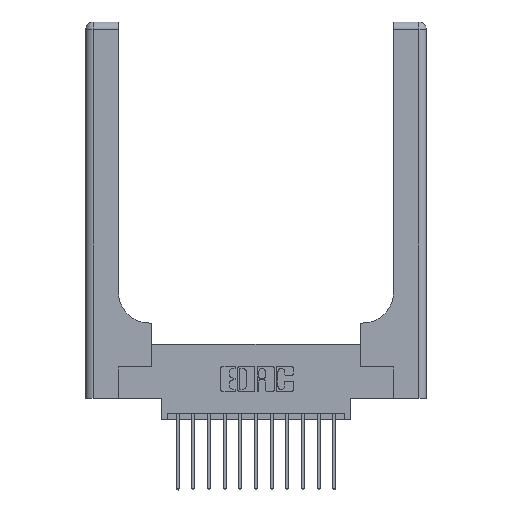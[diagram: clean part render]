
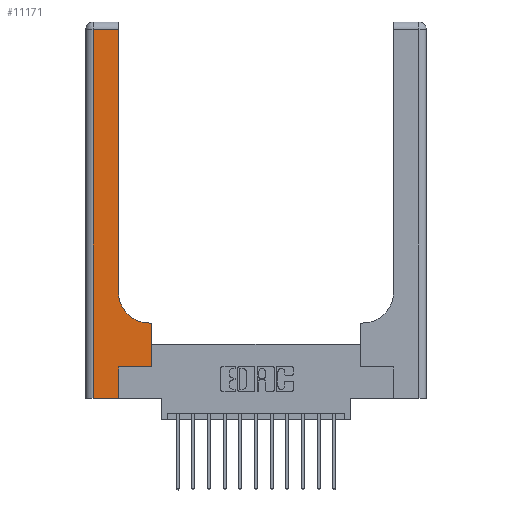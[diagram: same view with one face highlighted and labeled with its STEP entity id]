
A CAD part, top view. The second image highlights one B-rep face of the part: STEP entity #11171.
In plain terms, the highlighted planar face has unit normal (0, 0, 1).
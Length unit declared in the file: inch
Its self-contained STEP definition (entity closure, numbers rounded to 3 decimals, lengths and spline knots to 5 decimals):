
#109 = VERTEX_POINT ( 'NONE', #3793 ) ;
#213 = EDGE_CURVE ( 'NONE', #13001, #943, #8197, .T. ) ;
#262 = DIRECTION ( 'NONE',  ( -1., 0., 0. ) ) ;
#943 = VERTEX_POINT ( 'NONE', #5482 ) ;
#963 = CARTESIAN_POINT ( 'NONE',  ( 0.51, 0.85, 0.37 ) ) ;
#1099 = EDGE_CURVE ( 'NONE', #4193, #4466, #6357, .T. ) ;
#1140 = EDGE_CURVE ( 'NONE', #2775, #6244, #15808, .T. ) ;
#1279 = CARTESIAN_POINT ( 'NONE',  ( 0.51, 0.6, 0.37 ) ) ;
#1644 = DIRECTION ( 'NONE',  ( 0., 1., 0. ) ) ;
#2395 = CARTESIAN_POINT ( 'NONE',  ( 0.26, 2.94, 0.37 ) ) ;
#2755 = VECTOR ( 'NONE', #1644, 39.37008 ) ;
#2763 = AXIS2_PLACEMENT_3D ( 'NONE', #3532, #7427, #16393 ) ;
#2775 = VERTEX_POINT ( 'NONE', #16197 ) ;
#2839 = VERTEX_POINT ( 'NONE', #12482 ) ;
#2862 = CARTESIAN_POINT ( 'NONE',  ( 0., 0., 0.37 ) ) ;
#2903 = LINE ( 'NONE', #15711, #12800 ) ;
#2958 = ORIENTED_EDGE ( 'NONE', *, *, #14963, .T. ) ;
#3028 = LINE ( 'NONE', #16153, #12521 ) ;
#3342 = DIRECTION ( 'NONE',  ( -1., 0., 0. ) ) ;
#3440 = DIRECTION ( 'NONE',  ( 0., -1., 0. ) ) ;
#3529 = LINE ( 'NONE', #12420, #10009 ) ;
#3532 = CARTESIAN_POINT ( 'NONE',  ( 0., 3., 0.37 ) ) ;
#3559 = ORIENTED_EDGE ( 'NONE', *, *, #7947, .T. ) ;
#3599 = EDGE_LOOP ( 'NONE', ( #11252, #15025, #9006, #2958, #10245, #4564, #4969, #3559, #14855 ) ) ;
#3749 = EDGE_CURVE ( 'NONE', #6244, #2839, #3529, .T. ) ;
#3793 = CARTESIAN_POINT ( 'NONE',  ( 0.528, 0.6, 0.37 ) ) ;
#4193 = VERTEX_POINT ( 'NONE', #9388 ) ;
#4281 = VECTOR ( 'NONE', #10608, 39.37008 ) ;
#4339 = CARTESIAN_POINT ( 'NONE',  ( 0.528, 0.25, 0.37 ) ) ;
#4466 = VERTEX_POINT ( 'NONE', #7750 ) ;
#4563 = EDGE_CURVE ( 'NONE', #14065, #4193, #2903, .T. ) ;
#4564 = ORIENTED_EDGE ( 'NONE', *, *, #3749, .T. ) ;
#4969 = ORIENTED_EDGE ( 'NONE', *, *, #12594, .T. ) ;
#5482 = CARTESIAN_POINT ( 'NONE',  ( 0.26, 0.85, 0.37 ) ) ;
#5555 = DIRECTION ( 'NONE',  ( 0., 1., 0. ) ) ;
#6182 = LINE ( 'NONE', #4339, #2755 ) ;
#6244 = VERTEX_POINT ( 'NONE', #11823 ) ;
#6357 = LINE ( 'NONE', #9893, #12441 ) ;
#6841 = CARTESIAN_POINT ( 'NONE',  ( 0.26, 3., 0.37 ) ) ;
#7427 = DIRECTION ( 'NONE',  ( 0., 0., -1. ) ) ;
#7750 = CARTESIAN_POINT ( 'NONE',  ( 0.06, 0., 0.37 ) ) ;
#7947 = EDGE_CURVE ( 'NONE', #109, #13001, #3028, .T. ) ;
#8197 = CIRCLE ( 'NONE', #15819, 0.25 ) ;
#8573 = VECTOR ( 'NONE', #11255, 39.37008 ) ;
#8621 = CARTESIAN_POINT ( 'NONE',  ( 0.265, 0., 0.37 ) ) ;
#9006 = ORIENTED_EDGE ( 'NONE', *, *, #1099, .T. ) ;
#9269 = FACE_OUTER_BOUND ( 'NONE', #3599, .T. ) ;
#9388 = CARTESIAN_POINT ( 'NONE',  ( 0.06, 2.94, 0.37 ) ) ;
#9893 = CARTESIAN_POINT ( 'NONE',  ( 0.06, 3., 0.37 ) ) ;
#10009 = VECTOR ( 'NONE', #13679, 39.37008 ) ;
#10245 = ORIENTED_EDGE ( 'NONE', *, *, #1140, .T. ) ;
#10608 = DIRECTION ( 'NONE',  ( 1., 0., 0. ) ) ;
#11171 = ADVANCED_FACE ( 'NONE', ( #9269 ), #11285, .F. ) ;
#11252 = ORIENTED_EDGE ( 'NONE', *, *, #13751, .T. ) ;
#11255 = DIRECTION ( 'NONE',  ( 0., 1., 0. ) ) ;
#11285 = PLANE ( 'NONE',  #2763 ) ;
#11823 = CARTESIAN_POINT ( 'NONE',  ( 0.265, 0.25, 0.37 ) ) ;
#12420 = CARTESIAN_POINT ( 'NONE',  ( 0.265, 0.25, 0.37 ) ) ;
#12441 = VECTOR ( 'NONE', #3440, 39.37008 ) ;
#12482 = CARTESIAN_POINT ( 'NONE',  ( 0.528, 0.25, 0.37 ) ) ;
#12521 = VECTOR ( 'NONE', #3342, 39.37008 ) ;
#12594 = EDGE_CURVE ( 'NONE', #2839, #109, #6182, .T. ) ;
#12800 = VECTOR ( 'NONE', #262, 39.37008 ) ;
#13001 = VERTEX_POINT ( 'NONE', #1279 ) ;
#13621 = LINE ( 'NONE', #6841, #16602 ) ;
#13679 = DIRECTION ( 'NONE',  ( 1., 0., 0. ) ) ;
#13751 = EDGE_CURVE ( 'NONE', #943, #14065, #13621, .T. ) ;
#14065 = VERTEX_POINT ( 'NONE', #2395 ) ;
#14159 = LINE ( 'NONE', #2862, #4281 ) ;
#14855 = ORIENTED_EDGE ( 'NONE', *, *, #213, .T. ) ;
#14963 = EDGE_CURVE ( 'NONE', #4466, #2775, #14159, .T. ) ;
#15025 = ORIENTED_EDGE ( 'NONE', *, *, #4563, .T. ) ;
#15711 = CARTESIAN_POINT ( 'NONE',  ( 0., 2.94, 0.37 ) ) ;
#15808 = LINE ( 'NONE', #8621, #8573 ) ;
#15819 = AXIS2_PLACEMENT_3D ( 'NONE', #963, #16133, #16112 ) ;
#16112 = DIRECTION ( 'NONE',  ( 1., 0., 0. ) ) ;
#16133 = DIRECTION ( 'NONE',  ( 0., 0., -1. ) ) ;
#16153 = CARTESIAN_POINT ( 'NONE',  ( 0.26, 0.6, 0.37 ) ) ;
#16197 = CARTESIAN_POINT ( 'NONE',  ( 0.265, 0., 0.37 ) ) ;
#16393 = DIRECTION ( 'NONE',  ( -1., 0., 0. ) ) ;
#16602 = VECTOR ( 'NONE', #5555, 39.37008 ) ;
